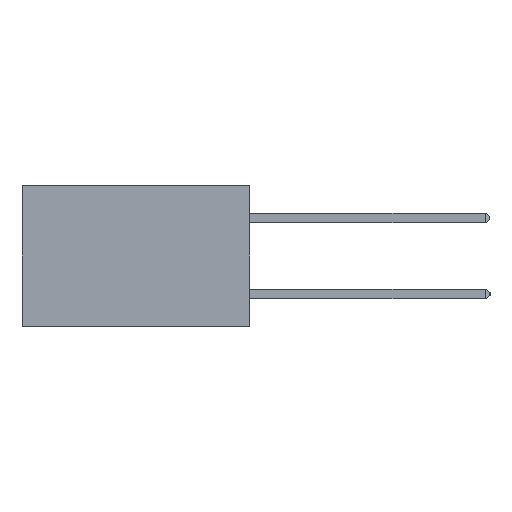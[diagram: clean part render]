
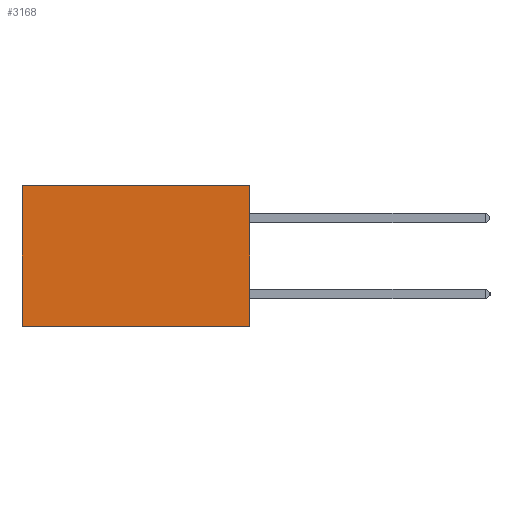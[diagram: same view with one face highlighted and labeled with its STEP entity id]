
A CAD part, left-side view. The second image highlights one B-rep face of the part: STEP entity #3168.
In plain terms, the highlighted planar face has unit normal (-1, 0, 0).
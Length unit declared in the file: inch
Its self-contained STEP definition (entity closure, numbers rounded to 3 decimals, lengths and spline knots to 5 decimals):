
#532 = LINE ( 'NONE', #12542, #10865 ) ;
#998 = EDGE_LOOP ( 'NONE', ( #6661, #4673, #12556, #1691 ) ) ;
#1198 = DIRECTION ( 'NONE',  ( 0., 0., -1. ) ) ;
#1691 = ORIENTED_EDGE ( 'NONE', *, *, #8803, .T. ) ;
#2030 = DIRECTION ( 'NONE',  ( 0., 1., 0. ) ) ;
#2443 = CARTESIAN_POINT ( 'NONE',  ( 0.2875, 0.6, 0. ) ) ;
#2939 = CARTESIAN_POINT ( 'NONE',  ( 0.2875, 0., 0. ) ) ;
#3168 = ADVANCED_FACE ( 'NONE', ( #11708 ), #10275, .F. ) ;
#3666 = CARTESIAN_POINT ( 'NONE',  ( 0.2875, 0., -0.37 ) ) ;
#3862 = EDGE_CURVE ( 'NONE', #10907, #6975, #532, .T. ) ;
#4673 = ORIENTED_EDGE ( 'NONE', *, *, #5117, .F. ) ;
#5117 = EDGE_CURVE ( 'NONE', #12319, #6975, #10679, .T. ) ;
#5194 = LINE ( 'NONE', #11889, #10443 ) ;
#5271 = DIRECTION ( 'NONE',  ( 1., 0., 0. ) ) ;
#5653 = AXIS2_PLACEMENT_3D ( 'NONE', #10326, #5271, #1198 ) ;
#6661 = ORIENTED_EDGE ( 'NONE', *, *, #3862, .T. ) ;
#6975 = VERTEX_POINT ( 'NONE', #13036 ) ;
#8254 = LINE ( 'NONE', #2939, #8910 ) ;
#8555 = CARTESIAN_POINT ( 'NONE',  ( 0.2875, 0., 0. ) ) ;
#8803 = EDGE_CURVE ( 'NONE', #9563, #10907, #5194, .T. ) ;
#8910 = VECTOR ( 'NONE', #9133, 39.37008 ) ;
#9133 = DIRECTION ( 'NONE',  ( 0., 0., -1. ) ) ;
#9433 = EDGE_CURVE ( 'NONE', #9563, #12319, #8254, .T. ) ;
#9563 = VERTEX_POINT ( 'NONE', #8555 ) ;
#10275 = PLANE ( 'NONE',  #5653 ) ;
#10326 = CARTESIAN_POINT ( 'NONE',  ( 0.2875, 0., 0. ) ) ;
#10443 = VECTOR ( 'NONE', #11935, 39.37008 ) ;
#10493 = DIRECTION ( 'NONE',  ( 0., 0., -1. ) ) ;
#10679 = LINE ( 'NONE', #12164, #12961 ) ;
#10865 = VECTOR ( 'NONE', #10493, 39.37008 ) ;
#10907 = VERTEX_POINT ( 'NONE', #2443 ) ;
#11708 = FACE_OUTER_BOUND ( 'NONE', #998, .T. ) ;
#11889 = CARTESIAN_POINT ( 'NONE',  ( 0.2875, 0., 0. ) ) ;
#11935 = DIRECTION ( 'NONE',  ( 0., 1., 0. ) ) ;
#12164 = CARTESIAN_POINT ( 'NONE',  ( 0.2875, 0., -0.37 ) ) ;
#12319 = VERTEX_POINT ( 'NONE', #3666 ) ;
#12542 = CARTESIAN_POINT ( 'NONE',  ( 0.2875, 0.6, 0. ) ) ;
#12556 = ORIENTED_EDGE ( 'NONE', *, *, #9433, .F. ) ;
#12961 = VECTOR ( 'NONE', #2030, 39.37008 ) ;
#13036 = CARTESIAN_POINT ( 'NONE',  ( 0.2875, 0.6, -0.37 ) ) ;
